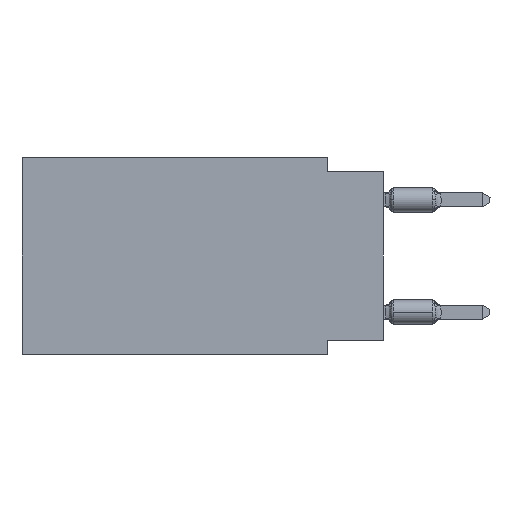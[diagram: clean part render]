
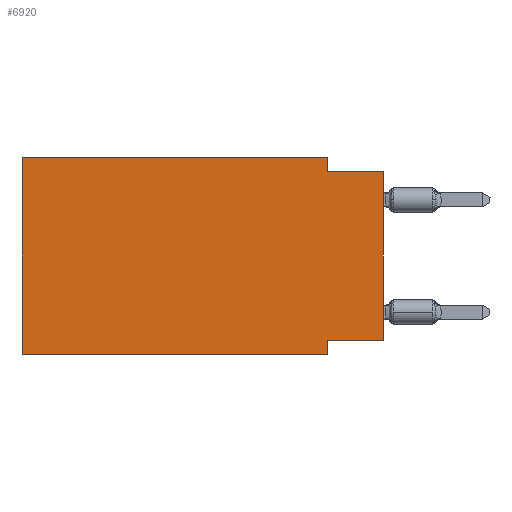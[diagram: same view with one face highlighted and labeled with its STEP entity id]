
A CAD part, left-side view. The second image highlights one B-rep face of the part: STEP entity #6920.
In plain terms, the highlighted planar face has unit normal (-1, 0, 0).
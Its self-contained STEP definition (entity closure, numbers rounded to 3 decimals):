
#903 = VECTOR ( 'NONE', #28274, 1000. ) ;
#1926 = ORIENTED_EDGE ( 'NONE', *, *, #45978, .T. ) ;
#4085 = EDGE_CURVE ( 'NONE', #18857, #16323, #16004, .T. ) ;
#4185 = EDGE_CURVE ( 'NONE', #32448, #23777, #44130, .T. ) ;
#4853 = CARTESIAN_POINT ( 'NONE',  ( 0., 2.54, 0. ) ) ;
#4981 = VERTEX_POINT ( 'NONE', #20405 ) ;
#6920 = ADVANCED_FACE ( 'NONE', ( #29997 ), #10545, .F. ) ;
#8374 = CARTESIAN_POINT ( 'NONE',  ( 0., 0., -0.635 ) ) ;
#8498 = VERTEX_POINT ( 'NONE', #11249 ) ;
#8697 = LINE ( 'NONE', #4853, #37014 ) ;
#9643 = LINE ( 'NONE', #29350, #33076 ) ;
#9731 = ORIENTED_EDGE ( 'NONE', *, *, #25843, .F. ) ;
#10545 = PLANE ( 'NONE',  #25629 ) ;
#10735 = VECTOR ( 'NONE', #15246, 1000. ) ;
#10922 = EDGE_LOOP ( 'NONE', ( #1926, #14626, #39703, #44654, #46607, #34915, #37804, #9731 ) ) ;
#11249 = CARTESIAN_POINT ( 'NONE',  ( 0., 2.54, -8.255 ) ) ;
#12948 = VECTOR ( 'NONE', #14827, 1000. ) ;
#13342 = CARTESIAN_POINT ( 'NONE',  ( 0., 0., -8.255 ) ) ;
#14626 = ORIENTED_EDGE ( 'NONE', *, *, #4085, .F. ) ;
#14827 = DIRECTION ( 'NONE',  ( 0., -1., 0. ) ) ;
#15246 = DIRECTION ( 'NONE',  ( 0., -1., 0. ) ) ;
#16004 = LINE ( 'NONE', #39551, #10735 ) ;
#16323 = VERTEX_POINT ( 'NONE', #8374 ) ;
#16698 = DIRECTION ( 'NONE',  ( 0., 0., -1. ) ) ;
#17320 = CARTESIAN_POINT ( 'NONE',  ( 0., 16.383, 0. ) ) ;
#17577 = DIRECTION ( 'NONE',  ( 0., 0., 1. ) ) ;
#18857 = VERTEX_POINT ( 'NONE', #27790 ) ;
#18983 = DIRECTION ( 'NONE',  ( 1., 0., 0. ) ) ;
#20033 = EDGE_CURVE ( 'NONE', #33796, #23057, #22508, .T. ) ;
#20286 = LINE ( 'NONE', #24626, #37650 ) ;
#20405 = CARTESIAN_POINT ( 'NONE',  ( 0., 0., -8.255 ) ) ;
#22508 = LINE ( 'NONE', #49907, #12948 ) ;
#22956 = LINE ( 'NONE', #30883, #47882 ) ;
#23057 = VERTEX_POINT ( 'NONE', #40492 ) ;
#23777 = VERTEX_POINT ( 'NONE', #34535 ) ;
#24554 = DIRECTION ( 'NONE',  ( 0., 0., -1. ) ) ;
#24626 = CARTESIAN_POINT ( 'NONE',  ( 0., 2.54, -8.89 ) ) ;
#25629 = AXIS2_PLACEMENT_3D ( 'NONE', #37948, #18983, #26915 ) ;
#25843 = EDGE_CURVE ( 'NONE', #4981, #8498, #48682, .T. ) ;
#26915 = DIRECTION ( 'NONE',  ( 0., 0., -1. ) ) ;
#27790 = CARTESIAN_POINT ( 'NONE',  ( 0., 2.54, -0.635 ) ) ;
#27824 = CARTESIAN_POINT ( 'NONE',  ( 0., 16.383, -8.89 ) ) ;
#28274 = DIRECTION ( 'NONE',  ( 0., -1., 0. ) ) ;
#29350 = CARTESIAN_POINT ( 'NONE',  ( 0., 0., 0. ) ) ;
#29997 = FACE_OUTER_BOUND ( 'NONE', #10922, .T. ) ;
#30883 = CARTESIAN_POINT ( 'NONE',  ( 0., 16.383, 0. ) ) ;
#32448 = VERTEX_POINT ( 'NONE', #17320 ) ;
#33052 = EDGE_CURVE ( 'NONE', #8498, #23057, #20286, .T. ) ;
#33076 = VECTOR ( 'NONE', #17577, 1000. ) ;
#33796 = VERTEX_POINT ( 'NONE', #27824 ) ;
#34535 = CARTESIAN_POINT ( 'NONE',  ( 0., 2.54, 0. ) ) ;
#34915 = ORIENTED_EDGE ( 'NONE', *, *, #20033, .T. ) ;
#37014 = VECTOR ( 'NONE', #24554, 1000. ) ;
#37228 = VECTOR ( 'NONE', #45088, 1000. ) ;
#37650 = VECTOR ( 'NONE', #16698, 1000. ) ;
#37804 = ORIENTED_EDGE ( 'NONE', *, *, #33052, .F. ) ;
#37948 = CARTESIAN_POINT ( 'NONE',  ( 0., 16.383, 0. ) ) ;
#39551 = CARTESIAN_POINT ( 'NONE',  ( 0., 0., -0.635 ) ) ;
#39703 = ORIENTED_EDGE ( 'NONE', *, *, #39916, .F. ) ;
#39916 = EDGE_CURVE ( 'NONE', #23777, #18857, #8697, .T. ) ;
#40492 = CARTESIAN_POINT ( 'NONE',  ( 0., 2.54, -8.89 ) ) ;
#40786 = CARTESIAN_POINT ( 'NONE',  ( 0., 16.383, 0. ) ) ;
#44130 = LINE ( 'NONE', #40786, #903 ) ;
#44654 = ORIENTED_EDGE ( 'NONE', *, *, #4185, .F. ) ;
#45088 = DIRECTION ( 'NONE',  ( 0., 1., 0. ) ) ;
#45978 = EDGE_CURVE ( 'NONE', #4981, #16323, #9643, .T. ) ;
#46607 = ORIENTED_EDGE ( 'NONE', *, *, #48557, .F. ) ;
#46771 = DIRECTION ( 'NONE',  ( 0., 0., 1. ) ) ;
#47882 = VECTOR ( 'NONE', #46771, 1000. ) ;
#48557 = EDGE_CURVE ( 'NONE', #33796, #32448, #22956, .T. ) ;
#48682 = LINE ( 'NONE', #13342, #37228 ) ;
#49907 = CARTESIAN_POINT ( 'NONE',  ( 0., 16.383, -8.89 ) ) ;
